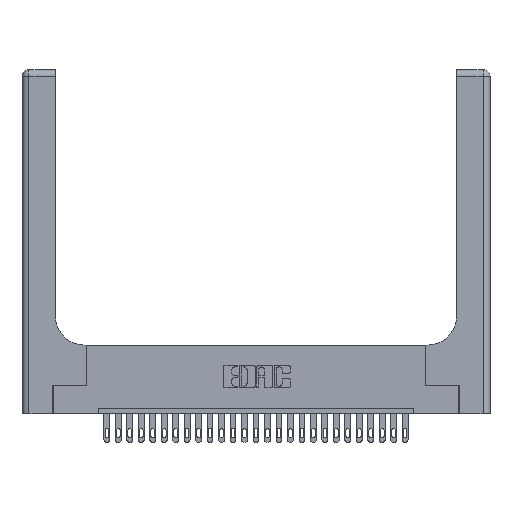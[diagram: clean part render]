
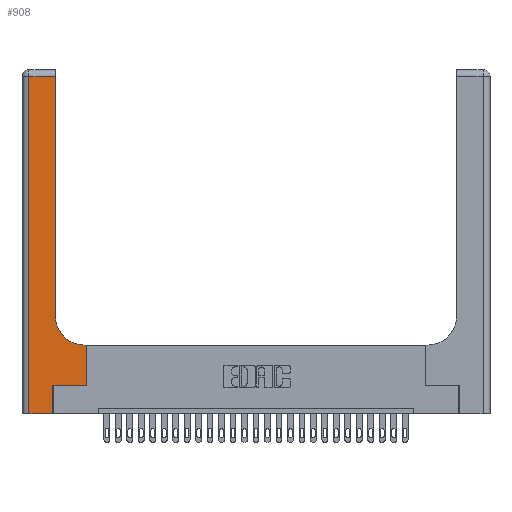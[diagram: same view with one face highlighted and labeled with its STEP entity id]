
A CAD part, top view. The second image highlights one B-rep face of the part: STEP entity #908.
In plain terms, the highlighted planar face has unit normal (0, 0, 1).
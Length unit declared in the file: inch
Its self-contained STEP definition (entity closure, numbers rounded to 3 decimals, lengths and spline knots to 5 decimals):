
#98 = CARTESIAN_POINT ( 'NONE',  ( 0.06, 0., 0.37 ) ) ;
#249 = VECTOR ( 'NONE', #7290, 39.37008 ) ;
#768 = CARTESIAN_POINT ( 'NONE',  ( 0.2915, 3., 0.37 ) ) ;
#908 = ADVANCED_FACE ( 'NONE', ( #6711 ), #16778, .F. ) ;
#1065 = CARTESIAN_POINT ( 'NONE',  ( 0., 2.94, 0.37 ) ) ;
#1477 = DIRECTION ( 'NONE',  ( 1., 0., 0. ) ) ;
#1624 = DIRECTION ( 'NONE',  ( 0., 0., -1. ) ) ;
#2019 = DIRECTION ( 'NONE',  ( 1., 0., 0. ) ) ;
#3147 = EDGE_CURVE ( 'NONE', #6020, #10048, #8863, .T. ) ;
#3156 = VECTOR ( 'NONE', #2019, 39.37008 ) ;
#3162 = ORIENTED_EDGE ( 'NONE', *, *, #18369, .T. ) ;
#3555 = EDGE_CURVE ( 'NONE', #14591, #27169, #4547, .T. ) ;
#4077 = CARTESIAN_POINT ( 'NONE',  ( 0., 3., 0.37 ) ) ;
#4497 = CARTESIAN_POINT ( 'NONE',  ( 0.2915, 2.94, 0.37 ) ) ;
#4537 = VERTEX_POINT ( 'NONE', #10506 ) ;
#4547 = LINE ( 'NONE', #1065, #249 ) ;
#5174 = EDGE_CURVE ( 'NONE', #8306, #14591, #25715, .T. ) ;
#5408 = VECTOR ( 'NONE', #1477, 39.37008 ) ;
#5844 = CARTESIAN_POINT ( 'NONE',  ( 0.269, 0.25, 0.37 ) ) ;
#6020 = VERTEX_POINT ( 'NONE', #21808 ) ;
#6290 = CARTESIAN_POINT ( 'NONE',  ( 0.2915, 0.6, 0.37 ) ) ;
#6711 = FACE_OUTER_BOUND ( 'NONE', #9025, .T. ) ;
#7290 = DIRECTION ( 'NONE',  ( -1., 0., 0. ) ) ;
#7577 = LINE ( 'NONE', #6290, #26134 ) ;
#7946 = DIRECTION ( 'NONE',  ( 0., 1., 0. ) ) ;
#8228 = CARTESIAN_POINT ( 'NONE',  ( 0.2915, 0.85, 0.37 ) ) ;
#8306 = VERTEX_POINT ( 'NONE', #8228 ) ;
#8863 = LINE ( 'NONE', #11896, #16536 ) ;
#8927 = LINE ( 'NONE', #13970, #26528 ) ;
#8961 = VERTEX_POINT ( 'NONE', #98 ) ;
#9025 = EDGE_LOOP ( 'NONE', ( #19922, #11500, #19219, #16404, #3162, #14248, #20350, #16024, #14573 ) ) ;
#9315 = CARTESIAN_POINT ( 'NONE',  ( 0.06, 2.94, 0.37 ) ) ;
#9739 = CIRCLE ( 'NONE', #22420, 0.25 ) ;
#10048 = VERTEX_POINT ( 'NONE', #10176 ) ;
#10176 = CARTESIAN_POINT ( 'NONE',  ( 0.5585, 0.6, 0.37 ) ) ;
#10310 = CARTESIAN_POINT ( 'NONE',  ( 0., 0., 0.37 ) ) ;
#10506 = CARTESIAN_POINT ( 'NONE',  ( 0.5415, 0.6, 0.37 ) ) ;
#10667 = VERTEX_POINT ( 'NONE', #5844 ) ;
#10712 = CARTESIAN_POINT ( 'NONE',  ( 0.269, 0., 0.37 ) ) ;
#11500 = ORIENTED_EDGE ( 'NONE', *, *, #3555, .T. ) ;
#11678 = LINE ( 'NONE', #24499, #22988 ) ;
#11798 = DIRECTION ( 'NONE',  ( 0., -1., 0. ) ) ;
#11896 = CARTESIAN_POINT ( 'NONE',  ( 0.5585, 0.25, 0.37 ) ) ;
#13970 = CARTESIAN_POINT ( 'NONE',  ( 0.269, 0., 0.37 ) ) ;
#14147 = CARTESIAN_POINT ( 'NONE',  ( 0.269, 0.25, 0.37 ) ) ;
#14248 = ORIENTED_EDGE ( 'NONE', *, *, #27230, .T. ) ;
#14341 = DIRECTION ( 'NONE',  ( 0., 0., -1. ) ) ;
#14379 = CARTESIAN_POINT ( 'NONE',  ( 0.5415, 0.85, 0.37 ) ) ;
#14424 = DIRECTION ( 'NONE',  ( -1., 0., 0. ) ) ;
#14573 = ORIENTED_EDGE ( 'NONE', *, *, #15050, .T. ) ;
#14591 = VERTEX_POINT ( 'NONE', #4497 ) ;
#15050 = EDGE_CURVE ( 'NONE', #4537, #8306, #9739, .T. ) ;
#15408 = VECTOR ( 'NONE', #18198, 39.37008 ) ;
#16024 = ORIENTED_EDGE ( 'NONE', *, *, #19794, .T. ) ;
#16036 = EDGE_CURVE ( 'NONE', #27169, #8961, #11678, .T. ) ;
#16404 = ORIENTED_EDGE ( 'NONE', *, *, #22633, .T. ) ;
#16532 = DIRECTION ( 'NONE',  ( 1., 0., 0. ) ) ;
#16536 = VECTOR ( 'NONE', #7946, 39.37008 ) ;
#16778 = PLANE ( 'NONE',  #18648 ) ;
#16851 = VERTEX_POINT ( 'NONE', #10712 ) ;
#18066 = LINE ( 'NONE', #10310, #3156 ) ;
#18198 = DIRECTION ( 'NONE',  ( 0., 1., 0. ) ) ;
#18369 = EDGE_CURVE ( 'NONE', #16851, #10667, #8927, .T. ) ;
#18648 = AXIS2_PLACEMENT_3D ( 'NONE', #4077, #14341, #14424 ) ;
#19129 = DIRECTION ( 'NONE',  ( -1., 0., 0. ) ) ;
#19219 = ORIENTED_EDGE ( 'NONE', *, *, #16036, .T. ) ;
#19794 = EDGE_CURVE ( 'NONE', #10048, #4537, #7577, .T. ) ;
#19922 = ORIENTED_EDGE ( 'NONE', *, *, #5174, .T. ) ;
#20350 = ORIENTED_EDGE ( 'NONE', *, *, #3147, .T. ) ;
#21808 = CARTESIAN_POINT ( 'NONE',  ( 0.5585, 0.25, 0.37 ) ) ;
#22420 = AXIS2_PLACEMENT_3D ( 'NONE', #14379, #1624, #16532 ) ;
#22633 = EDGE_CURVE ( 'NONE', #8961, #16851, #18066, .T. ) ;
#22988 = VECTOR ( 'NONE', #11798, 39.37008 ) ;
#24499 = CARTESIAN_POINT ( 'NONE',  ( 0.06, 3., 0.37 ) ) ;
#25279 = LINE ( 'NONE', #14147, #5408 ) ;
#25715 = LINE ( 'NONE', #768, #15408 ) ;
#26134 = VECTOR ( 'NONE', #19129, 39.37008 ) ;
#26528 = VECTOR ( 'NONE', #26758, 39.37008 ) ;
#26758 = DIRECTION ( 'NONE',  ( 0., 1., 0. ) ) ;
#27169 = VERTEX_POINT ( 'NONE', #9315 ) ;
#27230 = EDGE_CURVE ( 'NONE', #10667, #6020, #25279, .T. ) ;
